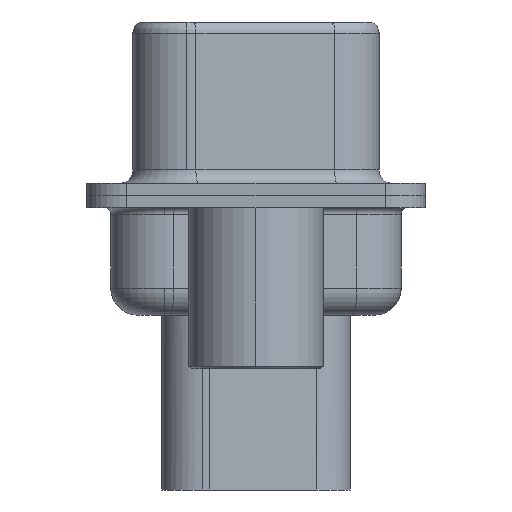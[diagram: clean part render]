
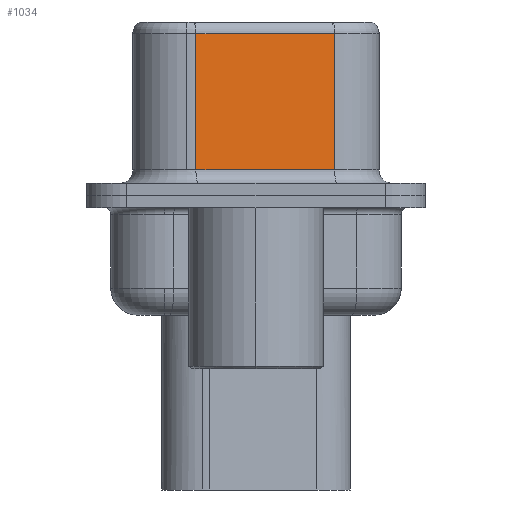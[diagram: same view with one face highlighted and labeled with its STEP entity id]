
A CAD part, left-side view. The second image highlights one B-rep face of the part: STEP entity #1034.
In plain terms, the highlighted planar face has unit normal (-0.985, -0.174, 0).
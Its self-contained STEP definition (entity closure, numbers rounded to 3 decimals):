
#261 = VECTOR ( 'NONE', #21442, 1000. ) ;
#1034 = ADVANCED_FACE ( 'NONE', ( #22548 ), #3003, .F. ) ;
#1064 = ORIENTED_EDGE ( 'NONE', *, *, #7076, .T. ) ;
#1141 = CARTESIAN_POINT ( 'NONE',  ( 4.58, -2.927, 0.95 ) ) ;
#2100 = DIRECTION ( 'NONE',  ( 0., 0., -1. ) ) ;
#3003 = PLANE ( 'NONE',  #5962 ) ;
#3222 = EDGE_CURVE ( 'NONE', #13742, #21207, #21086, .T. ) ;
#3706 = CARTESIAN_POINT ( 'NONE',  ( 4.58, -2.927, 6.52 ) ) ;
#4157 = CARTESIAN_POINT ( 'NONE',  ( 4.58, -2.927, 6.02 ) ) ;
#5962 = AXIS2_PLACEMENT_3D ( 'NONE', #11854, #20826, #15534 ) ;
#6674 = VECTOR ( 'NONE', #2100, 1000. ) ;
#7076 = EDGE_CURVE ( 'NONE', #7175, #13742, #9127, .T. ) ;
#7175 = VERTEX_POINT ( 'NONE', #21996 ) ;
#9042 = ORIENTED_EDGE ( 'NONE', *, *, #14107, .F. ) ;
#9127 = LINE ( 'NONE', #15795, #261 ) ;
#9274 = VECTOR ( 'NONE', #17515, 1000. ) ;
#11854 = CARTESIAN_POINT ( 'NONE',  ( 4.58, -2.927, 6.52 ) ) ;
#12774 = LINE ( 'NONE', #3706, #6674 ) ;
#13624 = EDGE_CURVE ( 'NONE', #19417, #7175, #16380, .T. ) ;
#13742 = VERTEX_POINT ( 'NONE', #20270 ) ;
#13958 = VECTOR ( 'NONE', #19817, 1000. ) ;
#14107 = EDGE_CURVE ( 'NONE', #19417, #21207, #12774, .T. ) ;
#15534 = DIRECTION ( 'NONE',  ( -0.174, 0.985, 0. ) ) ;
#15795 = CARTESIAN_POINT ( 'NONE',  ( 3.67, 2.233, 6.52 ) ) ;
#16380 = LINE ( 'NONE', #16488, #13958 ) ;
#16488 = CARTESIAN_POINT ( 'NONE',  ( 4.58, -2.927, 6.02 ) ) ;
#17515 = DIRECTION ( 'NONE',  ( 0.174, -0.985, 0. ) ) ;
#18598 = CARTESIAN_POINT ( 'NONE',  ( 4.58, -2.927, 0.95 ) ) ;
#18907 = ORIENTED_EDGE ( 'NONE', *, *, #3222, .T. ) ;
#19296 = EDGE_LOOP ( 'NONE', ( #9042, #21181, #1064, #18907 ) ) ;
#19417 = VERTEX_POINT ( 'NONE', #4157 ) ;
#19817 = DIRECTION ( 'NONE',  ( -0.174, 0.985, 0. ) ) ;
#20270 = CARTESIAN_POINT ( 'NONE',  ( 3.67, 2.233, 0.95 ) ) ;
#20826 = DIRECTION ( 'NONE',  ( 0.985, 0.174, 0. ) ) ;
#21086 = LINE ( 'NONE', #18598, #9274 ) ;
#21181 = ORIENTED_EDGE ( 'NONE', *, *, #13624, .T. ) ;
#21207 = VERTEX_POINT ( 'NONE', #1141 ) ;
#21442 = DIRECTION ( 'NONE',  ( 0., 0., -1. ) ) ;
#21996 = CARTESIAN_POINT ( 'NONE',  ( 3.67, 2.233, 6.02 ) ) ;
#22548 = FACE_OUTER_BOUND ( 'NONE', #19296, .T. ) ;
